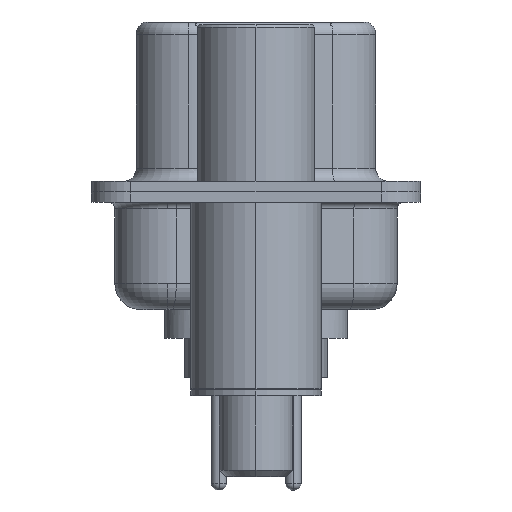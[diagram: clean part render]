
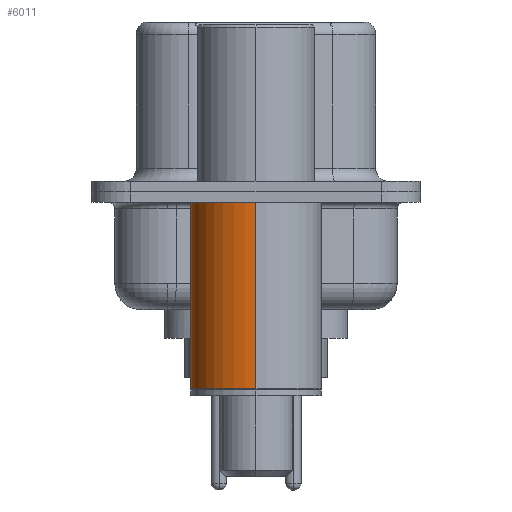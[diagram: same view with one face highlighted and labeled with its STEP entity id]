
A CAD part, left-side view. The second image highlights one B-rep face of the part: STEP entity #6011.
In plain terms, the highlighted cylindrical face has radius 2.5 mm (diameter 5 mm), a partial arc.
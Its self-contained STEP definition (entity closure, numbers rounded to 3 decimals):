
#616 = ORIENTED_EDGE ( 'NONE', *, *, #11535, .T. ) ;
#1701 = DIRECTION ( 'NONE',  ( 0., 0., 1. ) ) ;
#2260 = AXIS2_PLACEMENT_3D ( 'NONE', #10903, #11010, #11111 ) ;
#2334 = EDGE_LOOP ( 'NONE', ( #15737, #616, #28319, #20976 ) ) ;
#2789 = VECTOR ( 'NONE', #1701, 1000. ) ;
#4408 = CIRCLE ( 'NONE', #16814, 2.5 ) ;
#4908 = VERTEX_POINT ( 'NONE', #23651 ) ;
#6011 = ADVANCED_FACE ( 'NONE', ( #15508 ), #26844, .T. ) ;
#6153 = CARTESIAN_POINT ( 'NONE',  ( -2.5, 0., -7.525 ) ) ;
#6176 = CARTESIAN_POINT ( 'NONE',  ( 2.5, 0., 0.581 ) ) ;
#8718 = VERTEX_POINT ( 'NONE', #6153 ) ;
#9384 = CIRCLE ( 'NONE', #16169, 2.5 ) ;
#9952 = CARTESIAN_POINT ( 'NONE',  ( 0., 0., -7.525 ) ) ;
#10502 = CARTESIAN_POINT ( 'NONE',  ( 0., 0., -0.4 ) ) ;
#10903 = CARTESIAN_POINT ( 'NONE',  ( 0., 0., 0.581 ) ) ;
#11010 = DIRECTION ( 'NONE',  ( 0., 0., 1. ) ) ;
#11111 = DIRECTION ( 'NONE',  ( 1., 0., 0. ) ) ;
#11535 = EDGE_CURVE ( 'NONE', #8718, #4908, #27619, .T. ) ;
#12270 = DIRECTION ( 'NONE',  ( 1., 0., 0. ) ) ;
#12789 = DIRECTION ( 'NONE',  ( 1., 0., 0. ) ) ;
#13206 = DIRECTION ( 'NONE',  ( 0., 0., 1. ) ) ;
#14388 = VERTEX_POINT ( 'NONE', #20320 ) ;
#15508 = FACE_OUTER_BOUND ( 'NONE', #2334, .T. ) ;
#15737 = ORIENTED_EDGE ( 'NONE', *, *, #25185, .T. ) ;
#15821 = CARTESIAN_POINT ( 'NONE',  ( -2.5, 0., 0.581 ) ) ;
#16169 = AXIS2_PLACEMENT_3D ( 'NONE', #10502, #26766, #12789 ) ;
#16814 = AXIS2_PLACEMENT_3D ( 'NONE', #9952, #26236, #12270 ) ;
#18606 = LINE ( 'NONE', #6176, #24085 ) ;
#19953 = VERTEX_POINT ( 'NONE', #21748 ) ;
#20320 = CARTESIAN_POINT ( 'NONE',  ( 2.5, 0., -7.525 ) ) ;
#20976 = ORIENTED_EDGE ( 'NONE', *, *, #21511, .F. ) ;
#21511 = EDGE_CURVE ( 'NONE', #14388, #19953, #18606, .T. ) ;
#21748 = CARTESIAN_POINT ( 'NONE',  ( 2.5, 0., -0.4 ) ) ;
#23651 = CARTESIAN_POINT ( 'NONE',  ( -2.5, 0., -0.4 ) ) ;
#24085 = VECTOR ( 'NONE', #13206, 1000. ) ;
#25185 = EDGE_CURVE ( 'NONE', #14388, #8718, #4408, .T. ) ;
#26236 = DIRECTION ( 'NONE',  ( 0., 0., 1. ) ) ;
#26766 = DIRECTION ( 'NONE',  ( 0., 0., 1. ) ) ;
#26844 = CYLINDRICAL_SURFACE ( 'NONE', #2260, 2.5 ) ;
#27619 = LINE ( 'NONE', #15821, #2789 ) ;
#28319 = ORIENTED_EDGE ( 'NONE', *, *, #28370, .F. ) ;
#28370 = EDGE_CURVE ( 'NONE', #19953, #4908, #9384, .T. ) ;
